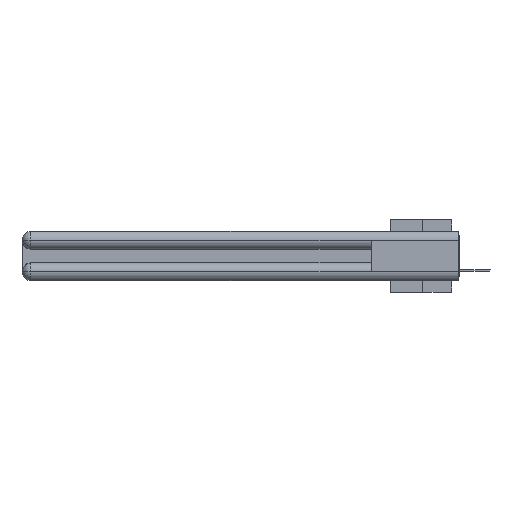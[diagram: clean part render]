
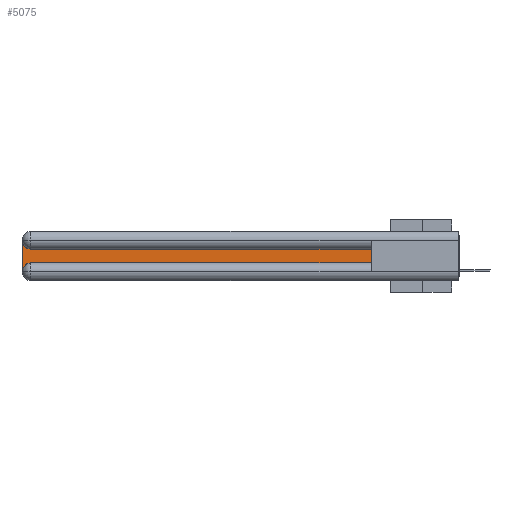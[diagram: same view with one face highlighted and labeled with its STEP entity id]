
A CAD part, left-side view. The second image highlights one B-rep face of the part: STEP entity #5075.
In plain terms, the highlighted planar face has unit normal (-1, 0, 0).
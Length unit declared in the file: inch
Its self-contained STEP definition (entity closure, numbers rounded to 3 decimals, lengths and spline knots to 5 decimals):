
#928 = CARTESIAN_POINT ( 'NONE',  ( 0.075, 0.6, -0.1225 ) ) ;
#957 = EDGE_CURVE ( 'NONE', #36550, #3391, #4773, .T. ) ;
#1548 = CARTESIAN_POINT ( 'NONE',  ( 0.075, 3., -0.2175 ) ) ;
#2707 = ORIENTED_EDGE ( 'NONE', *, *, #26235, .T. ) ;
#3391 = VERTEX_POINT ( 'NONE', #18447 ) ;
#4458 = VERTEX_POINT ( 'NONE', #28918 ) ;
#4738 = EDGE_LOOP ( 'NONE', ( #11234, #25547, #27241, #2707, #6218, #18106 ) ) ;
#4773 = LINE ( 'NONE', #1548, #14631 ) ;
#4985 = CIRCLE ( 'NONE', #17274, 0.06 ) ;
#5075 = ADVANCED_FACE ( 'NONE', ( #21126 ), #24167, .F. ) ;
#5746 = DIRECTION ( 'NONE',  ( 0., 0., 1. ) ) ;
#6218 = ORIENTED_EDGE ( 'NONE', *, *, #21998, .T. ) ;
#7191 = DIRECTION ( 'NONE',  ( 0., -1., 0. ) ) ;
#8396 = DIRECTION ( 'NONE',  ( 0., 0., -1. ) ) ;
#8735 = DIRECTION ( 'NONE',  ( 1., 0., 0. ) ) ;
#8762 = CARTESIAN_POINT ( 'NONE',  ( 0.075, 0.6, -0.2175 ) ) ;
#8981 = LINE ( 'NONE', #37180, #30124 ) ;
#9680 = LINE ( 'NONE', #28963, #18647 ) ;
#10081 = DIRECTION ( 'NONE',  ( 0., 1., 0. ) ) ;
#11094 = VERTEX_POINT ( 'NONE', #928 ) ;
#11234 = ORIENTED_EDGE ( 'NONE', *, *, #13771, .T. ) ;
#12290 = EDGE_CURVE ( 'NONE', #4458, #36550, #4985, .T. ) ;
#12292 = CARTESIAN_POINT ( 'NONE',  ( 0.075, 2.94, -0.0625 ) ) ;
#13771 = EDGE_CURVE ( 'NONE', #11094, #4458, #9680, .T. ) ;
#14323 = CARTESIAN_POINT ( 'NONE',  ( 0.075, 2.94, -0.2775 ) ) ;
#14631 = VECTOR ( 'NONE', #8396, 39.37008 ) ;
#15016 = CARTESIAN_POINT ( 'NONE',  ( 0.075, 3., -0.1225 ) ) ;
#17274 = AXIS2_PLACEMENT_3D ( 'NONE', #12292, #22033, #18976 ) ;
#17995 = VERTEX_POINT ( 'NONE', #8762 ) ;
#18106 = ORIENTED_EDGE ( 'NONE', *, *, #22345, .T. ) ;
#18447 = CARTESIAN_POINT ( 'NONE',  ( 0.075, 3., -0.2775 ) ) ;
#18483 = DIRECTION ( 'NONE',  ( 0., 0., -1. ) ) ;
#18647 = VECTOR ( 'NONE', #10081, 39.37008 ) ;
#18976 = DIRECTION ( 'NONE',  ( 0., 0., -1. ) ) ;
#19933 = AXIS2_PLACEMENT_3D ( 'NONE', #15016, #8735, #18483 ) ;
#19949 = CIRCLE ( 'NONE', #39352, 0.06 ) ;
#21126 = FACE_OUTER_BOUND ( 'NONE', #4738, .T. ) ;
#21998 = EDGE_CURVE ( 'NONE', #26283, #17995, #25864, .T. ) ;
#22033 = DIRECTION ( 'NONE',  ( 1., 0., 0. ) ) ;
#22345 = EDGE_CURVE ( 'NONE', #17995, #11094, #8981, .T. ) ;
#24167 = PLANE ( 'NONE',  #19933 ) ;
#25547 = ORIENTED_EDGE ( 'NONE', *, *, #12290, .T. ) ;
#25864 = LINE ( 'NONE', #35188, #32042 ) ;
#26235 = EDGE_CURVE ( 'NONE', #3391, #26283, #19949, .T. ) ;
#26283 = VERTEX_POINT ( 'NONE', #38693 ) ;
#27241 = ORIENTED_EDGE ( 'NONE', *, *, #957, .T. ) ;
#27489 = CARTESIAN_POINT ( 'NONE',  ( 0.075, 3., -0.0625 ) ) ;
#28918 = CARTESIAN_POINT ( 'NONE',  ( 0.075, 2.94, -0.1225 ) ) ;
#28963 = CARTESIAN_POINT ( 'NONE',  ( 0.075, 0.6, -0.1225 ) ) ;
#28974 = DIRECTION ( 'NONE',  ( 0., 0., -1. ) ) ;
#30124 = VECTOR ( 'NONE', #5746, 39.37008 ) ;
#32042 = VECTOR ( 'NONE', #7191, 39.37008 ) ;
#35060 = DIRECTION ( 'NONE',  ( 1., 0., 0. ) ) ;
#35188 = CARTESIAN_POINT ( 'NONE',  ( 0.075, 0.6, -0.2175 ) ) ;
#36550 = VERTEX_POINT ( 'NONE', #27489 ) ;
#37180 = CARTESIAN_POINT ( 'NONE',  ( 0.075, 0.6, -0.2175 ) ) ;
#38693 = CARTESIAN_POINT ( 'NONE',  ( 0.075, 2.94, -0.2175 ) ) ;
#39352 = AXIS2_PLACEMENT_3D ( 'NONE', #14323, #35060, #28974 ) ;
